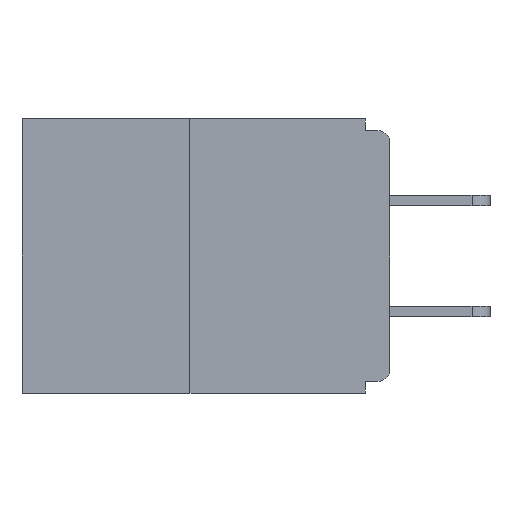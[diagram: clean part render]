
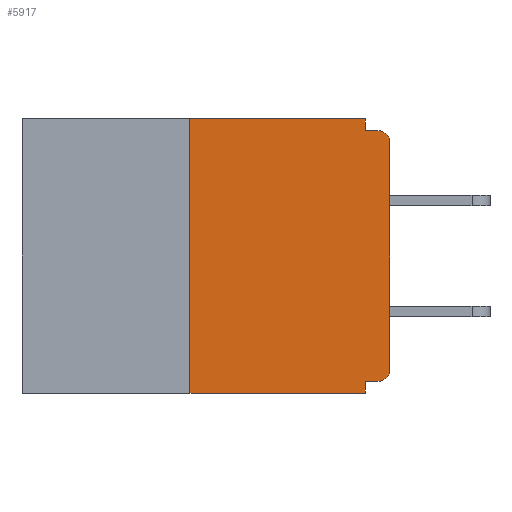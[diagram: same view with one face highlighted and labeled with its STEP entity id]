
A CAD part, left-side view. The second image highlights one B-rep face of the part: STEP entity #5917.
In plain terms, the highlighted planar face has unit normal (-1, 0, 0).
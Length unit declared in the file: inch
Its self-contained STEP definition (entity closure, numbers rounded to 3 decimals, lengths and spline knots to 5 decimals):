
#402 = LINE ( 'NONE', #19264, #6539 ) ;
#493 = CARTESIAN_POINT ( 'NONE',  ( 0., 0.46, 0. ) ) ;
#495 = DIRECTION ( 'NONE',  ( 0., 0., -1. ) ) ;
#626 = ORIENTED_EDGE ( 'NONE', *, *, #2677, .T. ) ;
#669 = CARTESIAN_POINT ( 'NONE',  ( 0., 0.46, 0. ) ) ;
#750 = CARTESIAN_POINT ( 'NONE',  ( 0., 0.031, 0. ) ) ;
#1202 = VERTEX_POINT ( 'NONE', #20744 ) ;
#1583 = EDGE_CURVE ( 'NONE', #13390, #10399, #14904, .T. ) ;
#2677 = EDGE_CURVE ( 'NONE', #16567, #15868, #17380, .T. ) ;
#2994 = AXIS2_PLACEMENT_3D ( 'NONE', #669, #6643, #495 ) ;
#3108 = EDGE_CURVE ( 'NONE', #8108, #15306, #24671, .T. ) ;
#3434 = VECTOR ( 'NONE', #22792, 39.37008 ) ;
#3461 = CARTESIAN_POINT ( 'NONE',  ( 0., 0.015, -0.313 ) ) ;
#3688 = CARTESIAN_POINT ( 'NONE',  ( 0., 0.031, -0.343 ) ) ;
#4955 = FACE_OUTER_BOUND ( 'NONE', #9424, .T. ) ;
#5184 = ORIENTED_EDGE ( 'NONE', *, *, #1583, .F. ) ;
#5613 = CARTESIAN_POINT ( 'NONE',  ( 0., 0., 0. ) ) ;
#5917 = ADVANCED_FACE ( 'NONE', ( #4955 ), #15060, .F. ) ;
#6029 = CARTESIAN_POINT ( 'NONE',  ( 0., 0., -0.03 ) ) ;
#6087 = DIRECTION ( 'NONE',  ( 0., 0., -1. ) ) ;
#6539 = VECTOR ( 'NONE', #23075, 39.37008 ) ;
#6643 = DIRECTION ( 'NONE',  ( 1., 0., 0. ) ) ;
#6663 = EDGE_CURVE ( 'NONE', #23123, #18584, #8601, .T. ) ;
#6830 = CARTESIAN_POINT ( 'NONE',  ( 0., 0.031, -0.343 ) ) ;
#8108 = VERTEX_POINT ( 'NONE', #19354 ) ;
#8297 = EDGE_CURVE ( 'NONE', #1202, #23443, #20150, .T. ) ;
#8601 = LINE ( 'NONE', #6830, #16683 ) ;
#8925 = LINE ( 'NONE', #20936, #3434 ) ;
#9367 = CARTESIAN_POINT ( 'NONE',  ( 0., 0., -0.015 ) ) ;
#9424 = EDGE_LOOP ( 'NONE', ( #26216, #10975, #12891, #21417, #24506, #13812, #13436, #626, #13528, #5184 ) ) ;
#9522 = EDGE_CURVE ( 'NONE', #1202, #18584, #402, .T. ) ;
#9767 = DIRECTION ( 'NONE',  ( 0., 0., 1. ) ) ;
#10399 = VERTEX_POINT ( 'NONE', #12472 ) ;
#10975 = ORIENTED_EDGE ( 'NONE', *, *, #8297, .F. ) ;
#11193 = VECTOR ( 'NONE', #20941, 39.37008 ) ;
#11393 = DIRECTION ( 'NONE',  ( 0., -1., 0. ) ) ;
#12051 = DIRECTION ( 'NONE',  ( 0., 0., 1. ) ) ;
#12472 = CARTESIAN_POINT ( 'NONE',  ( 0., 0.031, -0.015 ) ) ;
#12891 = ORIENTED_EDGE ( 'NONE', *, *, #9522, .T. ) ;
#12983 = LINE ( 'NONE', #5613, #19689 ) ;
#13006 = DIRECTION ( 'NONE',  ( 0., 0., -1. ) ) ;
#13390 = VERTEX_POINT ( 'NONE', #750 ) ;
#13436 = ORIENTED_EDGE ( 'NONE', *, *, #21809, .T. ) ;
#13528 = ORIENTED_EDGE ( 'NONE', *, *, #25004, .F. ) ;
#13605 = VECTOR ( 'NONE', #15759, 39.37008 ) ;
#13812 = ORIENTED_EDGE ( 'NONE', *, *, #3108, .T. ) ;
#14904 = LINE ( 'NONE', #15676, #13605 ) ;
#15060 = PLANE ( 'NONE',  #2994 ) ;
#15306 = VERTEX_POINT ( 'NONE', #21013 ) ;
#15549 = AXIS2_PLACEMENT_3D ( 'NONE', #3461, #17798, #19757 ) ;
#15676 = CARTESIAN_POINT ( 'NONE',  ( 0., 0.031, 0. ) ) ;
#15759 = DIRECTION ( 'NONE',  ( 0., 0., -1. ) ) ;
#15868 = VERTEX_POINT ( 'NONE', #22960 ) ;
#15899 = AXIS2_PLACEMENT_3D ( 'NONE', #24894, #16493, #6087 ) ;
#16086 = CARTESIAN_POINT ( 'NONE',  ( 0., 0.031, -0.328 ) ) ;
#16493 = DIRECTION ( 'NONE',  ( -1., 0., 0. ) ) ;
#16567 = VERTEX_POINT ( 'NONE', #6029 ) ;
#16683 = VECTOR ( 'NONE', #13006, 39.37008 ) ;
#17050 = EDGE_CURVE ( 'NONE', #8108, #23123, #8925, .T. ) ;
#17380 = CIRCLE ( 'NONE', #15899, 0.015 ) ;
#17798 = DIRECTION ( 'NONE',  ( -1., 0., 0. ) ) ;
#18584 = VERTEX_POINT ( 'NONE', #3688 ) ;
#19264 = CARTESIAN_POINT ( 'NONE',  ( 0., 0.46, -0.343 ) ) ;
#19354 = CARTESIAN_POINT ( 'NONE',  ( 0., 0.015, -0.328 ) ) ;
#19689 = VECTOR ( 'NONE', #9767, 39.37008 ) ;
#19757 = DIRECTION ( 'NONE',  ( 0., 0., -1. ) ) ;
#19812 = VECTOR ( 'NONE', #12051, 39.37008 ) ;
#20150 = LINE ( 'NONE', #24339, #19812 ) ;
#20499 = LINE ( 'NONE', #493, #11193 ) ;
#20744 = CARTESIAN_POINT ( 'NONE',  ( 0., 0.25, -0.343 ) ) ;
#20936 = CARTESIAN_POINT ( 'NONE',  ( 0., 0., -0.328 ) ) ;
#20941 = DIRECTION ( 'NONE',  ( 0., -1., 0. ) ) ;
#21013 = CARTESIAN_POINT ( 'NONE',  ( 0., 0., -0.313 ) ) ;
#21417 = ORIENTED_EDGE ( 'NONE', *, *, #6663, .F. ) ;
#21809 = EDGE_CURVE ( 'NONE', #15306, #16567, #12983, .T. ) ;
#22792 = DIRECTION ( 'NONE',  ( 0., 1., 0. ) ) ;
#22960 = CARTESIAN_POINT ( 'NONE',  ( 0., 0.015, -0.015 ) ) ;
#23075 = DIRECTION ( 'NONE',  ( 0., -1., 0. ) ) ;
#23123 = VERTEX_POINT ( 'NONE', #16086 ) ;
#23443 = VERTEX_POINT ( 'NONE', #25311 ) ;
#23912 = VECTOR ( 'NONE', #11393, 39.37008 ) ;
#24339 = CARTESIAN_POINT ( 'NONE',  ( 0., 0.25, 0. ) ) ;
#24506 = ORIENTED_EDGE ( 'NONE', *, *, #17050, .F. ) ;
#24567 = LINE ( 'NONE', #9367, #23912 ) ;
#24671 = CIRCLE ( 'NONE', #15549, 0.015 ) ;
#24894 = CARTESIAN_POINT ( 'NONE',  ( 0., 0.015, -0.03 ) ) ;
#25004 = EDGE_CURVE ( 'NONE', #10399, #15868, #24567, .T. ) ;
#25311 = CARTESIAN_POINT ( 'NONE',  ( 0., 0.25, 0. ) ) ;
#25929 = EDGE_CURVE ( 'NONE', #23443, #13390, #20499, .T. ) ;
#26216 = ORIENTED_EDGE ( 'NONE', *, *, #25929, .F. ) ;
